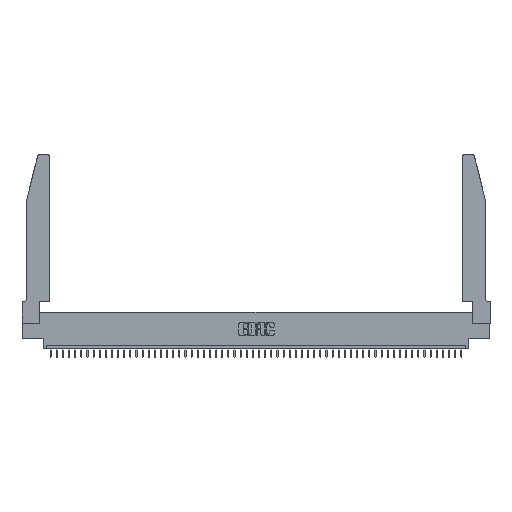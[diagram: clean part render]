
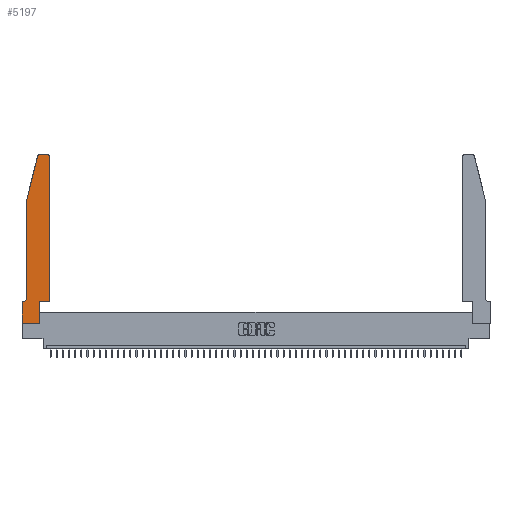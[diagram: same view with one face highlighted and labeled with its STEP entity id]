
A CAD part, top view. The second image highlights one B-rep face of the part: STEP entity #5197.
In plain terms, the highlighted planar face has unit normal (0, 0, 1).
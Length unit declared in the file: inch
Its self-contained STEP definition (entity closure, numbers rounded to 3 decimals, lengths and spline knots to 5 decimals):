
#766 = ORIENTED_EDGE ( 'NONE', *, *, #28183, .T. ) ;
#948 = CARTESIAN_POINT ( 'NONE',  ( 0.0755, 0.35, 0.37 ) ) ;
#1446 = VERTEX_POINT ( 'NONE', #29195 ) ;
#3135 = EDGE_CURVE ( 'NONE', #30482, #47074, #29402, .T. ) ;
#3510 = CARTESIAN_POINT ( 'NONE',  ( 0.2865, 0., 0.37 ) ) ;
#3851 = VECTOR ( 'NONE', #23522, 39.37008 ) ;
#4461 = CARTESIAN_POINT ( 'NONE',  ( 0., 0., 0.37 ) ) ;
#4750 = VERTEX_POINT ( 'NONE', #17110 ) ;
#5197 = ADVANCED_FACE ( 'NONE', ( #10451 ), #18956, .T. ) ;
#5515 = ORIENTED_EDGE ( 'NONE', *, *, #49440, .T. ) ;
#6626 = ORIENTED_EDGE ( 'NONE', *, *, #3135, .T. ) ;
#6658 = VERTEX_POINT ( 'NONE', #43542 ) ;
#7673 = CARTESIAN_POINT ( 'NONE',  ( 0.4505, 0.35, 0.37 ) ) ;
#8408 = DIRECTION ( 'NONE',  ( 1., 0., 0. ) ) ;
#8462 = DIRECTION ( 'NONE',  ( 1., 0., 0. ) ) ;
#8675 = DIRECTION ( 'NONE',  ( -1., 0., 0. ) ) ;
#8987 = VERTEX_POINT ( 'NONE', #10013 ) ;
#9242 = CIRCLE ( 'NONE', #31358, 0.07 ) ;
#9877 = LINE ( 'NONE', #22660, #13107 ) ;
#10013 = CARTESIAN_POINT ( 'NONE',  ( 0.4505, 0.35, 0.37 ) ) ;
#10451 = FACE_OUTER_BOUND ( 'NONE', #24473, .T. ) ;
#10663 = ORIENTED_EDGE ( 'NONE', *, *, #22138, .T. ) ;
#11272 = LINE ( 'NONE', #28041, #3851 ) ;
#12852 = ORIENTED_EDGE ( 'NONE', *, *, #50616, .T. ) ;
#13107 = VECTOR ( 'NONE', #22136, 39.37008 ) ;
#14158 = LINE ( 'NONE', #7673, #41073 ) ;
#14936 = DIRECTION ( 'NONE',  ( -0.239, -0.971, 0. ) ) ;
#15450 = ORIENTED_EDGE ( 'NONE', *, *, #22362, .T. ) ;
#15936 = DIRECTION ( 'NONE',  ( 0., 1., 0. ) ) ;
#16975 = CARTESIAN_POINT ( 'NONE',  ( 0., 0., 0.37 ) ) ;
#17110 = CARTESIAN_POINT ( 'NONE',  ( 0.4205, 2.75, 0.37 ) ) ;
#17189 = DIRECTION ( 'NONE',  ( 0., 0., 1. ) ) ;
#17798 = VERTEX_POINT ( 'NONE', #25561 ) ;
#17856 = DIRECTION ( 'NONE',  ( -1., 0., 0. ) ) ;
#18956 = PLANE ( 'NONE',  #35443 ) ;
#19658 = VERTEX_POINT ( 'NONE', #39307 ) ;
#19775 = EDGE_CURVE ( 'NONE', #42427, #42100, #20652, .T. ) ;
#19811 = EDGE_CURVE ( 'NONE', #19658, #45728, #29475, .T. ) ;
#20652 = LINE ( 'NONE', #948, #49021 ) ;
#21186 = DIRECTION ( 'NONE',  ( 0., 0., 1. ) ) ;
#21436 = CARTESIAN_POINT ( 'NONE',  ( 0.4205, 2.72, 0.37 ) ) ;
#22136 = DIRECTION ( 'NONE',  ( 0., -1., 0. ) ) ;
#22138 = EDGE_CURVE ( 'NONE', #4750, #19658, #33319, .T. ) ;
#22362 = EDGE_CURVE ( 'NONE', #17798, #42427, #9242, .T. ) ;
#22660 = CARTESIAN_POINT ( 'NONE',  ( 0.0755, 2., 0.37 ) ) ;
#22901 = CARTESIAN_POINT ( 'NONE',  ( 0.0055, 0.42, 0.37 ) ) ;
#22959 = DIRECTION ( 'NONE',  ( 0., 0., 1. ) ) ;
#23522 = DIRECTION ( 'NONE',  ( 1., 0., 0. ) ) ;
#24052 = EDGE_CURVE ( 'NONE', #42100, #1446, #28412, .T. ) ;
#24473 = EDGE_LOOP ( 'NONE', ( #10663, #26845, #5515, #52158, #15450, #48563, #51333, #766, #6626, #30154, #36180, #12852 ) ) ;
#25504 = LINE ( 'NONE', #4461, #49509 ) ;
#25561 = CARTESIAN_POINT ( 'NONE',  ( 0.0755, 0.42, 0.37 ) ) ;
#26416 = CARTESIAN_POINT ( 'NONE',  ( 0., 0.35, 0.37 ) ) ;
#26590 = AXIS2_PLACEMENT_3D ( 'NONE', #21436, #17189, #49942 ) ;
#26845 = ORIENTED_EDGE ( 'NONE', *, *, #19811, .T. ) ;
#28041 = CARTESIAN_POINT ( 'NONE',  ( 0.4505, 0.35, 0.37 ) ) ;
#28183 = EDGE_CURVE ( 'NONE', #1446, #30482, #25504, .T. ) ;
#28412 = LINE ( 'NONE', #16975, #31501 ) ;
#29043 = CARTESIAN_POINT ( 'NONE',  ( 0.2865, 0.35, 0.37 ) ) ;
#29195 = CARTESIAN_POINT ( 'NONE',  ( 0., 0., 0.37 ) ) ;
#29402 = LINE ( 'NONE', #42697, #36360 ) ;
#29475 = CIRCLE ( 'NONE', #38827, 0.03 ) ;
#30154 = ORIENTED_EDGE ( 'NONE', *, *, #41793, .T. ) ;
#30482 = VERTEX_POINT ( 'NONE', #3510 ) ;
#31358 = AXIS2_PLACEMENT_3D ( 'NONE', #22901, #39144, #51408 ) ;
#31501 = VECTOR ( 'NONE', #44133, 39.37008 ) ;
#31702 = CARTESIAN_POINT ( 'NONE',  ( 0.25487, 2.72718, 0.37 ) ) ;
#33319 = LINE ( 'NONE', #50346, #35594 ) ;
#34506 = CARTESIAN_POINT ( 'NONE',  ( 0.4505, 2.72, 0.37 ) ) ;
#35214 = CARTESIAN_POINT ( 'NONE',  ( 0., 0.35, 0.37 ) ) ;
#35443 = AXIS2_PLACEMENT_3D ( 'NONE', #35214, #22959, #43467 ) ;
#35594 = VECTOR ( 'NONE', #17856, 39.37008 ) ;
#36180 = ORIENTED_EDGE ( 'NONE', *, *, #51127, .T. ) ;
#36360 = VECTOR ( 'NONE', #41929, 39.37008 ) ;
#36383 = CARTESIAN_POINT ( 'NONE',  ( 0.284, 2.72, 0.37 ) ) ;
#38827 = AXIS2_PLACEMENT_3D ( 'NONE', #36383, #21186, #8408 ) ;
#39144 = DIRECTION ( 'NONE',  ( 0., 0., -1. ) ) ;
#39307 = CARTESIAN_POINT ( 'NONE',  ( 0.284, 2.75, 0.37 ) ) ;
#39728 = VERTEX_POINT ( 'NONE', #34506 ) ;
#40025 = EDGE_CURVE ( 'NONE', #6658, #17798, #9877, .T. ) ;
#41073 = VECTOR ( 'NONE', #15936, 39.37008 ) ;
#41793 = EDGE_CURVE ( 'NONE', #47074, #8987, #11272, .T. ) ;
#41929 = DIRECTION ( 'NONE',  ( 0., 1., 0. ) ) ;
#42100 = VERTEX_POINT ( 'NONE', #26416 ) ;
#42427 = VERTEX_POINT ( 'NONE', #45013 ) ;
#42697 = CARTESIAN_POINT ( 'NONE',  ( 0.2865, 0.35, 0.37 ) ) ;
#43467 = DIRECTION ( 'NONE',  ( 1., 0., 0. ) ) ;
#43542 = CARTESIAN_POINT ( 'NONE',  ( 0.0755, 2., 0.37 ) ) ;
#44133 = DIRECTION ( 'NONE',  ( 0., -1., 0. ) ) ;
#45013 = CARTESIAN_POINT ( 'NONE',  ( 0.0055, 0.35, 0.37 ) ) ;
#45728 = VERTEX_POINT ( 'NONE', #31702 ) ;
#46084 = VECTOR ( 'NONE', #14936, 39.37008 ) ;
#47074 = VERTEX_POINT ( 'NONE', #29043 ) ;
#47950 = LINE ( 'NONE', #52485, #46084 ) ;
#48563 = ORIENTED_EDGE ( 'NONE', *, *, #19775, .T. ) ;
#49021 = VECTOR ( 'NONE', #8675, 39.37008 ) ;
#49440 = EDGE_CURVE ( 'NONE', #45728, #6658, #47950, .T. ) ;
#49509 = VECTOR ( 'NONE', #8462, 39.37008 ) ;
#49942 = DIRECTION ( 'NONE',  ( 1., 0., 0. ) ) ;
#50346 = CARTESIAN_POINT ( 'NONE',  ( 0.2605, 2.75, 0.37 ) ) ;
#50616 = EDGE_CURVE ( 'NONE', #39728, #4750, #52088, .T. ) ;
#51127 = EDGE_CURVE ( 'NONE', #8987, #39728, #14158, .T. ) ;
#51333 = ORIENTED_EDGE ( 'NONE', *, *, #24052, .T. ) ;
#51408 = DIRECTION ( 'NONE',  ( -1., 0., 0. ) ) ;
#52088 = CIRCLE ( 'NONE', #26590, 0.03 ) ;
#52158 = ORIENTED_EDGE ( 'NONE', *, *, #40025, .T. ) ;
#52485 = CARTESIAN_POINT ( 'NONE',  ( 0.0755, 2., 0.37 ) ) ;
